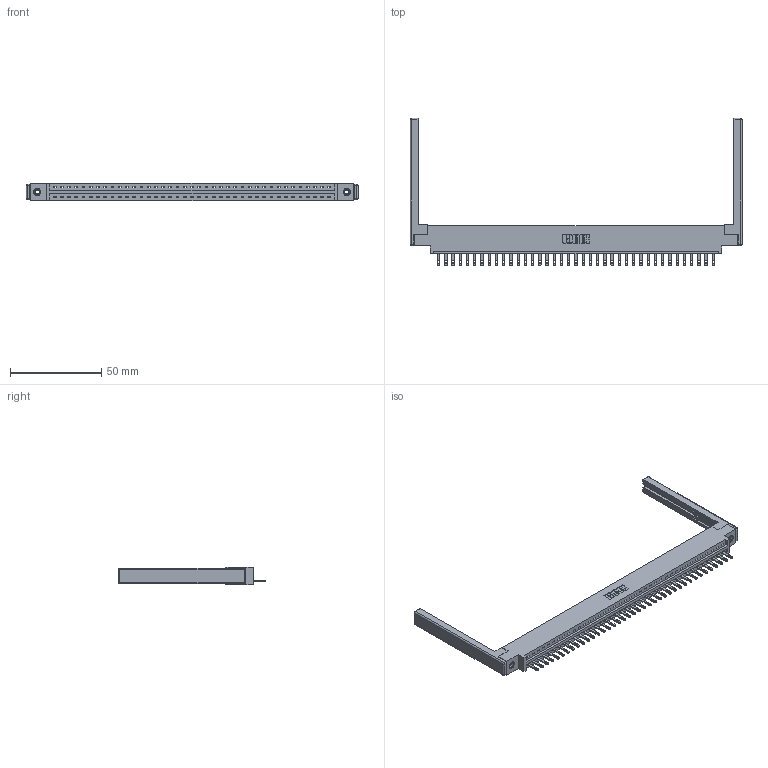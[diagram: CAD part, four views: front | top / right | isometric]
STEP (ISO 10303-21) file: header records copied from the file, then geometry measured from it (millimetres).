
FILE_DESCRIPTION (( 'STEP AP203' ), '1' );
FILE_NAME ('337-039-500-668.STEP', '2019-10-01T17:59:22', ( '' ), ( '' ), 'SwSTEP 2.0', 'SolidWorks 2016', '' );
FILE_SCHEMA (( 'CONFIG_CONTROL_DESIGN' ));
Length unit declared in the file: inch
Products named in the file (5): 337 Part_0.170 Offset - 0.156 Dia-TI; 345-292-001_345-293-100; 307-220-068; 337-039-500-668; 345-250-001_345-250-001-102
Assembly tree (44 placements, depth 2):
  337-039-500-668
    337 Part_0.170 Offset - 0.156 Dia-TI
    345-292-001_345-293-100  x39
    345-250-001_345-250-001-102  x2
    307-220-068  x2
Bounding box: 181.97 x 80.9 x 9.4 mm (x, y, z)
Volume: 23172.6 mm3; surface area: 23671.3 mm2
Topology: 44 solids, 44 shells, 2534 faces, 7733 edges, 5134 vertices
Faces by surface type: plane 1722, cylinder 788, cone 12, sphere 8, torus 4
Entity records: 32200 total; most frequent: CARTESIAN_POINT 5564, ORIENTED_EDGE 5528, DIRECTION 4764, EDGE_CURVE 2764, VECTOR 2582, LINE 2582, VERTEX_POINT 1834, AXIS2_PLACEMENT_3D 1091
